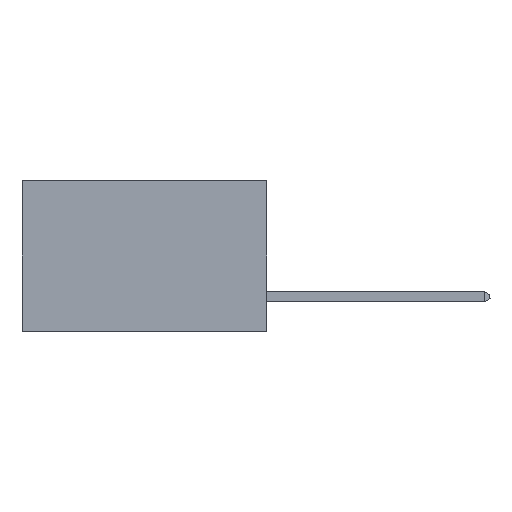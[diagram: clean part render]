
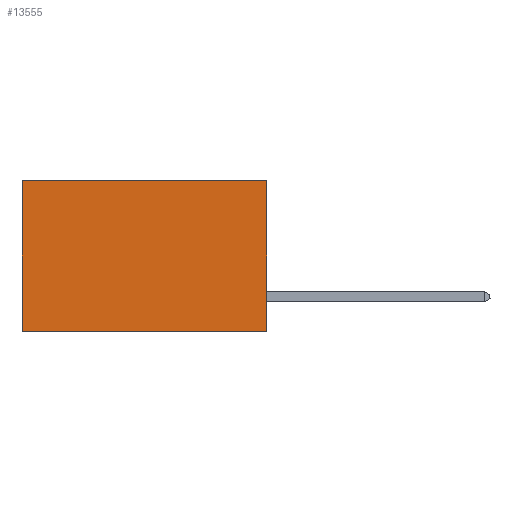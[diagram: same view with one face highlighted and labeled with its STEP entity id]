
A CAD part, left-side view. The second image highlights one B-rep face of the part: STEP entity #13555.
In plain terms, the highlighted planar face has unit normal (-1, 0, 0).
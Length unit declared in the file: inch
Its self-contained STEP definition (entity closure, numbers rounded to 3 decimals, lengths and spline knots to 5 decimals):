
#971 = EDGE_CURVE ( 'NONE', #14806, #5891, #31567, .T. ) ;
#3660 = VERTEX_POINT ( 'NONE', #11746 ) ;
#4233 = EDGE_CURVE ( 'NONE', #14806, #3660, #11978, .T. ) ;
#5658 = VECTOR ( 'NONE', #16501, 39.37008 ) ;
#5891 = VERTEX_POINT ( 'NONE', #27668 ) ;
#6421 = VECTOR ( 'NONE', #36147, 39.37008 ) ;
#7188 = VERTEX_POINT ( 'NONE', #24526 ) ;
#8435 = AXIS2_PLACEMENT_3D ( 'NONE', #21158, #30259, #13044 ) ;
#8568 = CARTESIAN_POINT ( 'NONE',  ( 0.2875, 0., 0. ) ) ;
#10463 = LINE ( 'NONE', #30161, #6421 ) ;
#10512 = ORIENTED_EDGE ( 'NONE', *, *, #35335, .F. ) ;
#11246 = FACE_OUTER_BOUND ( 'NONE', #15312, .T. ) ;
#11696 = ORIENTED_EDGE ( 'NONE', *, *, #971, .F. ) ;
#11746 = CARTESIAN_POINT ( 'NONE',  ( 0.2875, 0.6, 0. ) ) ;
#11978 = LINE ( 'NONE', #27905, #5658 ) ;
#12513 = DIRECTION ( 'NONE',  ( 0., 0., -1. ) ) ;
#13044 = DIRECTION ( 'NONE',  ( 0., 0., -1. ) ) ;
#13555 = ADVANCED_FACE ( 'NONE', ( #11246 ), #17728, .F. ) ;
#14806 = VERTEX_POINT ( 'NONE', #8568 ) ;
#15247 = VECTOR ( 'NONE', #12513, 39.37008 ) ;
#15312 = EDGE_LOOP ( 'NONE', ( #33962, #10512, #11696, #27031 ) ) ;
#16501 = DIRECTION ( 'NONE',  ( 0., 1., 0. ) ) ;
#16850 = DIRECTION ( 'NONE',  ( 0., 1., 0. ) ) ;
#17728 = PLANE ( 'NONE',  #8435 ) ;
#18199 = CARTESIAN_POINT ( 'NONE',  ( 0.2875, 0., 0. ) ) ;
#19354 = LINE ( 'NONE', #34108, #36103 ) ;
#21158 = CARTESIAN_POINT ( 'NONE',  ( 0.2875, 0., 0. ) ) ;
#24526 = CARTESIAN_POINT ( 'NONE',  ( 0.2875, 0.6, -0.37 ) ) ;
#27031 = ORIENTED_EDGE ( 'NONE', *, *, #4233, .T. ) ;
#27668 = CARTESIAN_POINT ( 'NONE',  ( 0.2875, 0., -0.37 ) ) ;
#27905 = CARTESIAN_POINT ( 'NONE',  ( 0.2875, 0., 0. ) ) ;
#29214 = EDGE_CURVE ( 'NONE', #3660, #7188, #10463, .T. ) ;
#30161 = CARTESIAN_POINT ( 'NONE',  ( 0.2875, 0.6, 0. ) ) ;
#30259 = DIRECTION ( 'NONE',  ( 1., 0., 0. ) ) ;
#31567 = LINE ( 'NONE', #18199, #15247 ) ;
#33962 = ORIENTED_EDGE ( 'NONE', *, *, #29214, .T. ) ;
#34108 = CARTESIAN_POINT ( 'NONE',  ( 0.2875, 0., -0.37 ) ) ;
#35335 = EDGE_CURVE ( 'NONE', #5891, #7188, #19354, .T. ) ;
#36103 = VECTOR ( 'NONE', #16850, 39.37008 ) ;
#36147 = DIRECTION ( 'NONE',  ( 0., 0., -1. ) ) ;
